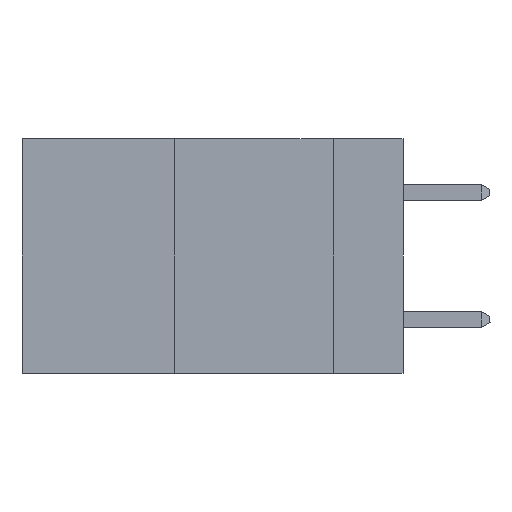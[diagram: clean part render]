
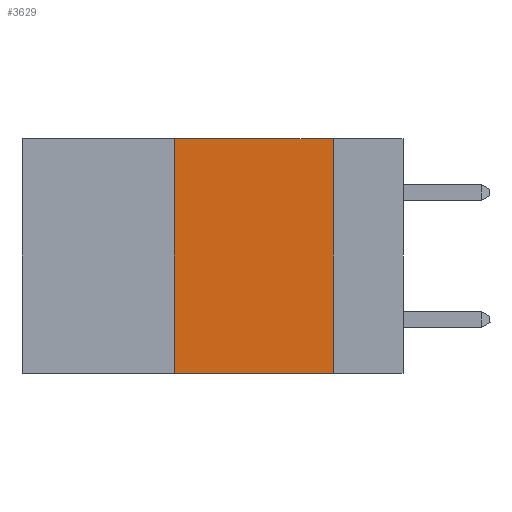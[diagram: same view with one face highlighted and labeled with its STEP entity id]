
A CAD part, left-side view. The second image highlights one B-rep face of the part: STEP entity #3629.
In plain terms, the highlighted planar face has unit normal (-1, 0, 0).
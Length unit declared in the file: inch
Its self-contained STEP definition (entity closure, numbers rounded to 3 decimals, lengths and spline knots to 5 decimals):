
#211 = ORIENTED_EDGE ( 'NONE', *, *, #960, .F. ) ;
#744 = ORIENTED_EDGE ( 'NONE', *, *, #18345, .F. ) ;
#960 = EDGE_CURVE ( 'NONE', #20914, #18265, #14831, .T. ) ;
#1406 = CARTESIAN_POINT ( 'NONE',  ( 0., 0.6, -0.37 ) ) ;
#2667 = DIRECTION ( 'NONE',  ( 0., 0., -1. ) ) ;
#2846 = PLANE ( 'NONE',  #10176 ) ;
#3629 = ADVANCED_FACE ( 'NONE', ( #16285 ), #2846, .F. ) ;
#4762 = CARTESIAN_POINT ( 'NONE',  ( 0., 0.11, 0. ) ) ;
#5851 = CARTESIAN_POINT ( 'NONE',  ( 0., 0.36, -0.37 ) ) ;
#7820 = DIRECTION ( 'NONE',  ( 0., -1., 0. ) ) ;
#9275 = DIRECTION ( 'NONE',  ( 0., -1., 0. ) ) ;
#9871 = LINE ( 'NONE', #12454, #17751 ) ;
#10176 = AXIS2_PLACEMENT_3D ( 'NONE', #21593, #15243, #2667 ) ;
#12454 = CARTESIAN_POINT ( 'NONE',  ( 0., 0.36, 0. ) ) ;
#13138 = CARTESIAN_POINT ( 'NONE',  ( 0., 0.11, 0. ) ) ;
#13865 = VECTOR ( 'NONE', #7820, 39.37008 ) ;
#14831 = LINE ( 'NONE', #4762, #17108 ) ;
#15243 = DIRECTION ( 'NONE',  ( 1., 0., 0. ) ) ;
#16285 = FACE_OUTER_BOUND ( 'NONE', #21942, .T. ) ;
#17108 = VECTOR ( 'NONE', #25571, 39.37008 ) ;
#17538 = CARTESIAN_POINT ( 'NONE',  ( 0., 0.6, 0. ) ) ;
#17751 = VECTOR ( 'NONE', #24917, 39.37008 ) ;
#18265 = VERTEX_POINT ( 'NONE', #21785 ) ;
#18345 = EDGE_CURVE ( 'NONE', #24853, #20914, #19269, .T. ) ;
#19258 = VERTEX_POINT ( 'NONE', #5851 ) ;
#19269 = LINE ( 'NONE', #17538, #25793 ) ;
#20574 = ORIENTED_EDGE ( 'NONE', *, *, #22471, .T. ) ;
#20830 = CARTESIAN_POINT ( 'NONE',  ( 0., 0.36, 0. ) ) ;
#20914 = VERTEX_POINT ( 'NONE', #13138 ) ;
#21593 = CARTESIAN_POINT ( 'NONE',  ( 0., 0.6, 0. ) ) ;
#21785 = CARTESIAN_POINT ( 'NONE',  ( 0., 0.11, -0.37 ) ) ;
#21942 = EDGE_LOOP ( 'NONE', ( #211, #744, #23485, #20574 ) ) ;
#22397 = LINE ( 'NONE', #1406, #13865 ) ;
#22471 = EDGE_CURVE ( 'NONE', #19258, #18265, #22397, .T. ) ;
#23148 = EDGE_CURVE ( 'NONE', #19258, #24853, #9871, .T. ) ;
#23485 = ORIENTED_EDGE ( 'NONE', *, *, #23148, .F. ) ;
#24853 = VERTEX_POINT ( 'NONE', #20830 ) ;
#24917 = DIRECTION ( 'NONE',  ( 0., 0., 1. ) ) ;
#25571 = DIRECTION ( 'NONE',  ( 0., 0., -1. ) ) ;
#25793 = VECTOR ( 'NONE', #9275, 39.37008 ) ;
